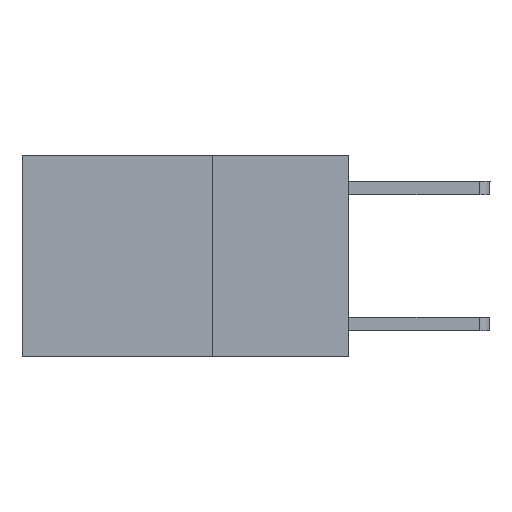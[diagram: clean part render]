
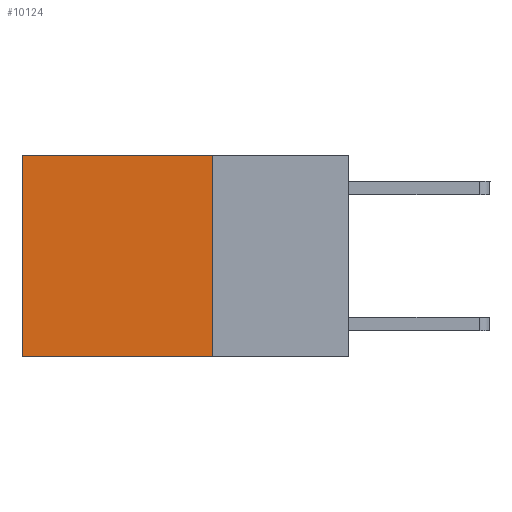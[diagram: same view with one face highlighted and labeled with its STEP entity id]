
A CAD part, left-side view. The second image highlights one B-rep face of the part: STEP entity #10124.
In plain terms, the highlighted planar face has unit normal (-1, 0, 0).
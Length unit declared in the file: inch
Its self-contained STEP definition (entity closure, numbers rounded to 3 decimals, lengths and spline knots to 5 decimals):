
#108 = ORIENTED_EDGE ( 'NONE', *, *, #5319, .F. ) ;
#455 = VECTOR ( 'NONE', #5771, 39.37008 ) ;
#654 = LINE ( 'NONE', #9165, #8246 ) ;
#794 = DIRECTION ( 'NONE',  ( 0., 0., -1. ) ) ;
#1340 = VERTEX_POINT ( 'NONE', #4214 ) ;
#1427 = LINE ( 'NONE', #5154, #7116 ) ;
#1502 = VERTEX_POINT ( 'NONE', #8623 ) ;
#1559 = EDGE_CURVE ( 'NONE', #1340, #9176, #7352, .T. ) ;
#1584 = CARTESIAN_POINT ( 'NONE',  ( 0.2625, 0.25, 0. ) ) ;
#1639 = FACE_OUTER_BOUND ( 'NONE', #5790, .T. ) ;
#2152 = CARTESIAN_POINT ( 'NONE',  ( 0.2625, 0.25, 0. ) ) ;
#2899 = DIRECTION ( 'NONE',  ( 0., 0., -1. ) ) ;
#3425 = ORIENTED_EDGE ( 'NONE', *, *, #5074, .T. ) ;
#4214 = CARTESIAN_POINT ( 'NONE',  ( 0.2625, 0.6, 0. ) ) ;
#4498 = CARTESIAN_POINT ( 'NONE',  ( 0.2625, 0.25, 0. ) ) ;
#5074 = EDGE_CURVE ( 'NONE', #7832, #1340, #9256, .T. ) ;
#5094 = AXIS2_PLACEMENT_3D ( 'NONE', #1584, #9519, #794 ) ;
#5154 = CARTESIAN_POINT ( 'NONE',  ( 0.2625, 0.25, 0. ) ) ;
#5319 = EDGE_CURVE ( 'NONE', #1502, #9176, #654, .T. ) ;
#5505 = PLANE ( 'NONE',  #5094 ) ;
#5771 = DIRECTION ( 'NONE',  ( 0., 0., -1. ) ) ;
#5790 = EDGE_LOOP ( 'NONE', ( #5797, #108, #8550, #3425 ) ) ;
#5797 = ORIENTED_EDGE ( 'NONE', *, *, #1559, .T. ) ;
#5818 = CARTESIAN_POINT ( 'NONE',  ( 0.2625, 0.6, 0. ) ) ;
#6748 = VECTOR ( 'NONE', #8477, 39.37008 ) ;
#6878 = EDGE_CURVE ( 'NONE', #7832, #1502, #1427, .T. ) ;
#6994 = DIRECTION ( 'NONE',  ( 0., 1., 0. ) ) ;
#7116 = VECTOR ( 'NONE', #2899, 39.37008 ) ;
#7352 = LINE ( 'NONE', #5818, #455 ) ;
#7832 = VERTEX_POINT ( 'NONE', #4498 ) ;
#8246 = VECTOR ( 'NONE', #6994, 39.37008 ) ;
#8303 = CARTESIAN_POINT ( 'NONE',  ( 0.2625, 0.6, -0.37 ) ) ;
#8477 = DIRECTION ( 'NONE',  ( 0., 1., 0. ) ) ;
#8550 = ORIENTED_EDGE ( 'NONE', *, *, #6878, .F. ) ;
#8623 = CARTESIAN_POINT ( 'NONE',  ( 0.2625, 0.25, -0.37 ) ) ;
#9165 = CARTESIAN_POINT ( 'NONE',  ( 0.2625, 0.25, -0.37 ) ) ;
#9176 = VERTEX_POINT ( 'NONE', #8303 ) ;
#9256 = LINE ( 'NONE', #2152, #6748 ) ;
#9519 = DIRECTION ( 'NONE',  ( 1., 0., 0. ) ) ;
#10124 = ADVANCED_FACE ( 'NONE', ( #1639 ), #5505, .F. ) ;
